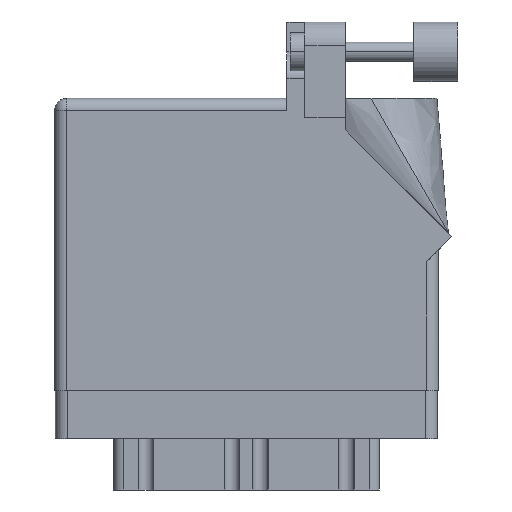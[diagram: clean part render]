
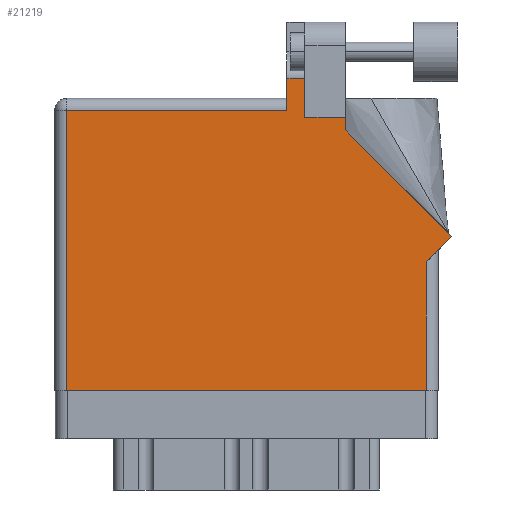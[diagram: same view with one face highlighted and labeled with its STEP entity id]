
A CAD part, front view. The second image highlights one B-rep face of the part: STEP entity #21219.
In plain terms, the highlighted face is planar.
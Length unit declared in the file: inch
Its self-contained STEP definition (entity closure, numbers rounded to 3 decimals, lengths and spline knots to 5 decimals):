
#58 = VERTEX_POINT ( 'NONE', #19266 ) ;
#1416 = EDGE_CURVE ( 'NONE', #10544, #58, #9366, .T. ) ;
#2051 = CARTESIAN_POINT ( 'NONE',  ( 0., 0., 0. ) ) ;
#2176 = ORIENTED_EDGE ( 'NONE', *, *, #30518, .T. ) ;
#2224 = EDGE_CURVE ( 'NONE', #29290, #19484, #17287, .T. ) ;
#2425 = CARTESIAN_POINT ( 'NONE',  ( 1.64177, 1.6315, 0. ) ) ;
#2925 = ORIENTED_EDGE ( 'NONE', *, *, #4004, .T. ) ;
#2934 = DIRECTION ( 'NONE',  ( 0., 1., 0. ) ) ;
#3083 = VERTEX_POINT ( 'NONE', #14437 ) ;
#3099 = CARTESIAN_POINT ( 'NONE',  ( 1.948, 0.675, 0. ) ) ;
#3166 = DIRECTION ( 'NONE',  ( -1., 0., 0. ) ) ;
#3771 = ORIENTED_EDGE ( 'NONE', *, *, #5338, .T. ) ;
#4004 = EDGE_CURVE ( 'NONE', #13395, #10544, #31077, .T. ) ;
#4382 = VECTOR ( 'NONE', #16887, 39.37008 ) ;
#4500 = LINE ( 'NONE', #21524, #24672 ) ;
#4578 = CARTESIAN_POINT ( 'NONE',  ( 0.062, 0., 0. ) ) ;
#5338 = EDGE_CURVE ( 'NONE', #23804, #21720, #24451, .T. ) ;
#6384 = LINE ( 'NONE', #28290, #29774 ) ;
#6396 = CARTESIAN_POINT ( 'NONE',  ( 1.524, 1.43, 0. ) ) ;
#7272 = CARTESIAN_POINT ( 'NONE',  ( 1.311, 1.43, 0. ) ) ;
#7745 = VECTOR ( 'NONE', #10753, 39.37008 ) ;
#7748 = CARTESIAN_POINT ( 'NONE',  ( 2.08071, 0.80771, 0. ) ) ;
#7868 = VERTEX_POINT ( 'NONE', #9001 ) ;
#7928 = AXIS2_PLACEMENT_3D ( 'NONE', #13153, #20723, #23246 ) ;
#8227 = CARTESIAN_POINT ( 'NONE',  ( 0.062, 1.468, 0. ) ) ;
#8691 = CARTESIAN_POINT ( 'NONE',  ( 1.948, 0., 0. ) ) ;
#9001 = CARTESIAN_POINT ( 'NONE',  ( 1.524, 1.36442, 0. ) ) ;
#9047 = EDGE_CURVE ( 'NONE', #58, #23804, #28086, .T. ) ;
#9366 = LINE ( 'NONE', #2425, #25798 ) ;
#10544 = VERTEX_POINT ( 'NONE', #30565 ) ;
#10753 = DIRECTION ( 'NONE',  ( 0., -1., 0. ) ) ;
#10789 = PLANE ( 'NONE',  #7928 ) ;
#11378 = CARTESIAN_POINT ( 'NONE',  ( 1.217, 1.53, 0. ) ) ;
#11869 = CARTESIAN_POINT ( 'NONE',  ( 1.217, 1.468, 0. ) ) ;
#12553 = CARTESIAN_POINT ( 'NONE',  ( 1.948, 0.737, 0. ) ) ;
#12932 = VERTEX_POINT ( 'NONE', #6396 ) ;
#13153 = CARTESIAN_POINT ( 'NONE',  ( 0., 1.53, 0. ) ) ;
#13395 = VERTEX_POINT ( 'NONE', #16443 ) ;
#13695 = VECTOR ( 'NONE', #15299, 39.37008 ) ;
#13945 = DIRECTION ( 'NONE',  ( 0.707, 0.707, 0. ) ) ;
#14148 = CARTESIAN_POINT ( 'NONE',  ( 1.524, 1.36442, 0. ) ) ;
#14200 = DIRECTION ( 'NONE',  ( 0., -1., 0. ) ) ;
#14437 = CARTESIAN_POINT ( 'NONE',  ( 0.062, 0., 0. ) ) ;
#15299 = DIRECTION ( 'NONE',  ( -1., 0., 0. ) ) ;
#16443 = CARTESIAN_POINT ( 'NONE',  ( 1.311, 1.43, 0. ) ) ;
#16887 = DIRECTION ( 'NONE',  ( 0., 1., 0. ) ) ;
#16924 = EDGE_CURVE ( 'NONE', #21720, #3083, #26164, .T. ) ;
#17287 = LINE ( 'NONE', #12553, #17783 ) ;
#17783 = VECTOR ( 'NONE', #31178, 39.37008 ) ;
#18860 = VECTOR ( 'NONE', #2934, 39.37008 ) ;
#18884 = LINE ( 'NONE', #14148, #18860 ) ;
#18958 = EDGE_LOOP ( 'NONE', ( #2925, #29897, #28899, #3771, #27784, #23884, #29270, #19535, #31074, #2176, #20535 ) ) ;
#19085 = EDGE_CURVE ( 'NONE', #3083, #29290, #23656, .T. ) ;
#19266 = CARTESIAN_POINT ( 'NONE',  ( 1.217, 1.6315, 0. ) ) ;
#19484 = VERTEX_POINT ( 'NONE', #3099 ) ;
#19535 = ORIENTED_EDGE ( 'NONE', *, *, #26212, .T. ) ;
#19711 = VERTEX_POINT ( 'NONE', #23899 ) ;
#20535 = ORIENTED_EDGE ( 'NONE', *, *, #23476, .T. ) ;
#20723 = DIRECTION ( 'NONE',  ( 0., 0., -1. ) ) ;
#21219 = ADVANCED_FACE ( 'NONE', ( #27492 ), #10789, .F. ) ;
#21524 = CARTESIAN_POINT ( 'NONE',  ( 1.524, 1.43, 0. ) ) ;
#21654 = VECTOR ( 'NONE', #14200, 39.37008 ) ;
#21720 = VERTEX_POINT ( 'NONE', #8227 ) ;
#22099 = LINE ( 'NONE', #7748, #26415 ) ;
#22542 = CARTESIAN_POINT ( 'NONE',  ( 0., 1.468, 0. ) ) ;
#23246 = DIRECTION ( 'NONE',  ( -1., 0., 0. ) ) ;
#23476 = EDGE_CURVE ( 'NONE', #12932, #13395, #4500, .T. ) ;
#23656 = LINE ( 'NONE', #2051, #24792 ) ;
#23804 = VERTEX_POINT ( 'NONE', #11869 ) ;
#23819 = DIRECTION ( 'NONE',  ( 1., 0., 0. ) ) ;
#23884 = ORIENTED_EDGE ( 'NONE', *, *, #19085, .T. ) ;
#23899 = CARTESIAN_POINT ( 'NONE',  ( 2.08071, 0.80771, 0. ) ) ;
#24451 = LINE ( 'NONE', #22542, #13695 ) ;
#24672 = VECTOR ( 'NONE', #30992, 39.37008 ) ;
#24792 = VECTOR ( 'NONE', #23819, 39.37008 ) ;
#24929 = DIRECTION ( 'NONE',  ( -0.707, 0.707, 0. ) ) ;
#25798 = VECTOR ( 'NONE', #3166, 39.37008 ) ;
#26164 = LINE ( 'NONE', #4578, #21654 ) ;
#26212 = EDGE_CURVE ( 'NONE', #19484, #19711, #6384, .T. ) ;
#26415 = VECTOR ( 'NONE', #24929, 39.37008 ) ;
#27492 = FACE_OUTER_BOUND ( 'NONE', #18958, .T. ) ;
#27784 = ORIENTED_EDGE ( 'NONE', *, *, #16924, .T. ) ;
#28086 = LINE ( 'NONE', #11378, #7745 ) ;
#28290 = CARTESIAN_POINT ( 'NONE',  ( 2.01, 0.737, 0. ) ) ;
#28899 = ORIENTED_EDGE ( 'NONE', *, *, #9047, .T. ) ;
#29270 = ORIENTED_EDGE ( 'NONE', *, *, #2224, .T. ) ;
#29290 = VERTEX_POINT ( 'NONE', #8691 ) ;
#29774 = VECTOR ( 'NONE', #13945, 39.37008 ) ;
#29897 = ORIENTED_EDGE ( 'NONE', *, *, #1416, .T. ) ;
#30518 = EDGE_CURVE ( 'NONE', #7868, #12932, #18884, .T. ) ;
#30565 = CARTESIAN_POINT ( 'NONE',  ( 1.311, 1.6315, 0. ) ) ;
#30955 = EDGE_CURVE ( 'NONE', #19711, #7868, #22099, .T. ) ;
#30992 = DIRECTION ( 'NONE',  ( -1., 0., 0. ) ) ;
#31074 = ORIENTED_EDGE ( 'NONE', *, *, #30955, .T. ) ;
#31077 = LINE ( 'NONE', #7272, #4382 ) ;
#31178 = DIRECTION ( 'NONE',  ( 0., 1., 0. ) ) ;
